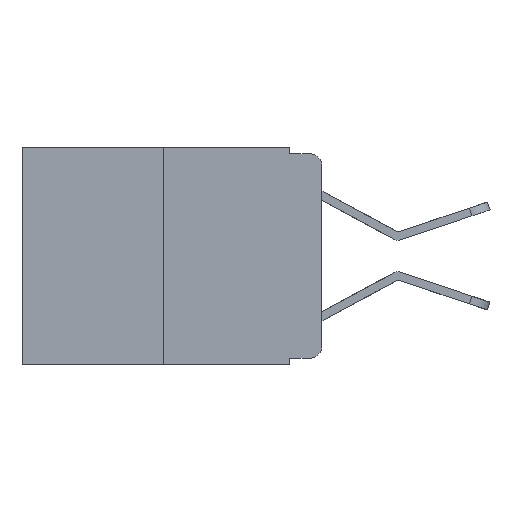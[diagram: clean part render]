
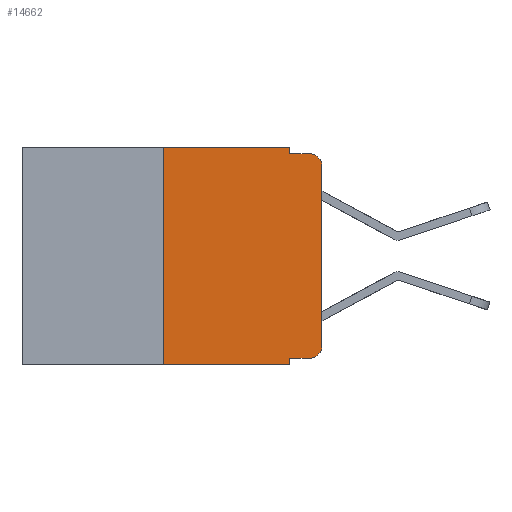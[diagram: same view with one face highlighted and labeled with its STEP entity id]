
A CAD part, left-side view. The second image highlights one B-rep face of the part: STEP entity #14662.
In plain terms, the highlighted planar face has unit normal (-1, 0, 0).
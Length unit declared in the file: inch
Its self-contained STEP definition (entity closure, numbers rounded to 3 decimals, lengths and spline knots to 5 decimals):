
#14 = EDGE_CURVE ( 'NONE', #7621, #17167, #16243, .T. ) ;
#318 = CARTESIAN_POINT ( 'NONE',  ( 0., 0.051, -0.333 ) ) ;
#724 = CARTESIAN_POINT ( 'NONE',  ( 0., 0.25, -0.343 ) ) ;
#845 = ORIENTED_EDGE ( 'NONE', *, *, #14, .F. ) ;
#1090 = CARTESIAN_POINT ( 'NONE',  ( 0., 0., -0.03 ) ) ;
#1284 = CARTESIAN_POINT ( 'NONE',  ( 0., 0.051, -0.343 ) ) ;
#1725 = CARTESIAN_POINT ( 'NONE',  ( 0., 0.051, -0.01 ) ) ;
#1763 = DIRECTION ( 'NONE',  ( 0., -1., 0. ) ) ;
#1811 = EDGE_CURVE ( 'NONE', #20390, #15506, #3043, .T. ) ;
#2113 = VECTOR ( 'NONE', #1763, 39.37008 ) ;
#2385 = AXIS2_PLACEMENT_3D ( 'NONE', #15543, #7231, #17490 ) ;
#3043 = CIRCLE ( 'NONE', #18014, 0.02 ) ;
#3376 = DIRECTION ( 'NONE',  ( 0., -1., 0. ) ) ;
#3629 = EDGE_CURVE ( 'NONE', #17167, #7439, #4998, .T. ) ;
#3699 = LINE ( 'NONE', #5309, #13990 ) ;
#3892 = DIRECTION ( 'NONE',  ( 0., 0., -1. ) ) ;
#4603 = AXIS2_PLACEMENT_3D ( 'NONE', #19205, #6649, #20706 ) ;
#4998 = LINE ( 'NONE', #14012, #7427 ) ;
#5215 = ORIENTED_EDGE ( 'NONE', *, *, #8182, .F. ) ;
#5258 = PLANE ( 'NONE',  #4603 ) ;
#5309 = CARTESIAN_POINT ( 'NONE',  ( 0., 0., 0. ) ) ;
#5416 = CARTESIAN_POINT ( 'NONE',  ( 0., 0., -0.313 ) ) ;
#5626 = DIRECTION ( 'NONE',  ( 0., 0., 1. ) ) ;
#5988 = DIRECTION ( 'NONE',  ( 0., -1., 0. ) ) ;
#6022 = EDGE_CURVE ( 'NONE', #21608, #20390, #3699, .T. ) ;
#6180 = ORIENTED_EDGE ( 'NONE', *, *, #15974, .F. ) ;
#6278 = CARTESIAN_POINT ( 'NONE',  ( 0., 0.051, 0. ) ) ;
#6649 = DIRECTION ( 'NONE',  ( 1., 0., 0. ) ) ;
#6947 = DIRECTION ( 'NONE',  ( 0., -1., 0. ) ) ;
#7139 = CIRCLE ( 'NONE', #2385, 0.02 ) ;
#7231 = DIRECTION ( 'NONE',  ( -1., 0., 0. ) ) ;
#7427 = VECTOR ( 'NONE', #3376, 39.37008 ) ;
#7439 = VERTEX_POINT ( 'NONE', #8085 ) ;
#7621 = VERTEX_POINT ( 'NONE', #724 ) ;
#8014 = LINE ( 'NONE', #6278, #8093 ) ;
#8085 = CARTESIAN_POINT ( 'NONE',  ( 0., 0.051, 0. ) ) ;
#8093 = VECTOR ( 'NONE', #20213, 39.37008 ) ;
#8182 = EDGE_CURVE ( 'NONE', #7439, #10505, #8014, .T. ) ;
#8303 = VECTOR ( 'NONE', #5626, 39.37008 ) ;
#9052 = DIRECTION ( 'NONE',  ( -1., 0., 0. ) ) ;
#9126 = CARTESIAN_POINT ( 'NONE',  ( 0., 0.25, 0. ) ) ;
#9324 = CARTESIAN_POINT ( 'NONE',  ( 0., 0.051, 0. ) ) ;
#10240 = VERTEX_POINT ( 'NONE', #17766 ) ;
#10256 = EDGE_LOOP ( 'NONE', ( #18085, #15320, #6180, #5215, #19069, #845, #22455, #16043, #18541, #10769 ) ) ;
#10505 = VERTEX_POINT ( 'NONE', #1725 ) ;
#10556 = CARTESIAN_POINT ( 'NONE',  ( 0., 0.051, -0.01 ) ) ;
#10769 = ORIENTED_EDGE ( 'NONE', *, *, #16571, .T. ) ;
#10903 = CARTESIAN_POINT ( 'NONE',  ( 0., 0.25, 0. ) ) ;
#11293 = EDGE_CURVE ( 'NONE', #22453, #10240, #17431, .T. ) ;
#11965 = VECTOR ( 'NONE', #21566, 39.37008 ) ;
#13901 = CARTESIAN_POINT ( 'NONE',  ( 0., 0.051, -0.333 ) ) ;
#13965 = EDGE_CURVE ( 'NONE', #7621, #19789, #17985, .T. ) ;
#13990 = VECTOR ( 'NONE', #17523, 39.37008 ) ;
#14012 = CARTESIAN_POINT ( 'NONE',  ( 0., 0.473, 0. ) ) ;
#14662 = ADVANCED_FACE ( 'NONE', ( #17135 ), #5258, .F. ) ;
#15320 = ORIENTED_EDGE ( 'NONE', *, *, #1811, .T. ) ;
#15452 = CARTESIAN_POINT ( 'NONE',  ( 0., 0.02, -0.01 ) ) ;
#15506 = VERTEX_POINT ( 'NONE', #15452 ) ;
#15543 = CARTESIAN_POINT ( 'NONE',  ( 0., 0.02, -0.313 ) ) ;
#15974 = EDGE_CURVE ( 'NONE', #10505, #15506, #20754, .T. ) ;
#16043 = ORIENTED_EDGE ( 'NONE', *, *, #22506, .F. ) ;
#16243 = LINE ( 'NONE', #10903, #8303 ) ;
#16571 = EDGE_CURVE ( 'NONE', #10240, #21608, #7139, .T. ) ;
#17135 = FACE_OUTER_BOUND ( 'NONE', #10256, .T. ) ;
#17167 = VERTEX_POINT ( 'NONE', #9126 ) ;
#17431 = LINE ( 'NONE', #13901, #19953 ) ;
#17490 = DIRECTION ( 'NONE',  ( 0., 0., -1. ) ) ;
#17523 = DIRECTION ( 'NONE',  ( 0., 0., 1. ) ) ;
#17766 = CARTESIAN_POINT ( 'NONE',  ( 0., 0.02, -0.333 ) ) ;
#17985 = LINE ( 'NONE', #21548, #18457 ) ;
#18005 = LINE ( 'NONE', #9324, #11965 ) ;
#18014 = AXIS2_PLACEMENT_3D ( 'NONE', #19795, #9052, #3892 ) ;
#18085 = ORIENTED_EDGE ( 'NONE', *, *, #6022, .T. ) ;
#18457 = VECTOR ( 'NONE', #5988, 39.37008 ) ;
#18541 = ORIENTED_EDGE ( 'NONE', *, *, #11293, .T. ) ;
#19069 = ORIENTED_EDGE ( 'NONE', *, *, #3629, .F. ) ;
#19205 = CARTESIAN_POINT ( 'NONE',  ( 0., 0.473, 0. ) ) ;
#19789 = VERTEX_POINT ( 'NONE', #1284 ) ;
#19795 = CARTESIAN_POINT ( 'NONE',  ( 0., 0.02, -0.03 ) ) ;
#19953 = VECTOR ( 'NONE', #6947, 39.37008 ) ;
#20213 = DIRECTION ( 'NONE',  ( 0., 0., -1. ) ) ;
#20390 = VERTEX_POINT ( 'NONE', #1090 ) ;
#20706 = DIRECTION ( 'NONE',  ( 0., 0., -1. ) ) ;
#20754 = LINE ( 'NONE', #10556, #2113 ) ;
#21548 = CARTESIAN_POINT ( 'NONE',  ( 0., 0.473, -0.343 ) ) ;
#21566 = DIRECTION ( 'NONE',  ( 0., 0., -1. ) ) ;
#21608 = VERTEX_POINT ( 'NONE', #5416 ) ;
#22453 = VERTEX_POINT ( 'NONE', #318 ) ;
#22455 = ORIENTED_EDGE ( 'NONE', *, *, #13965, .T. ) ;
#22506 = EDGE_CURVE ( 'NONE', #22453, #19789, #18005, .T. ) ;
